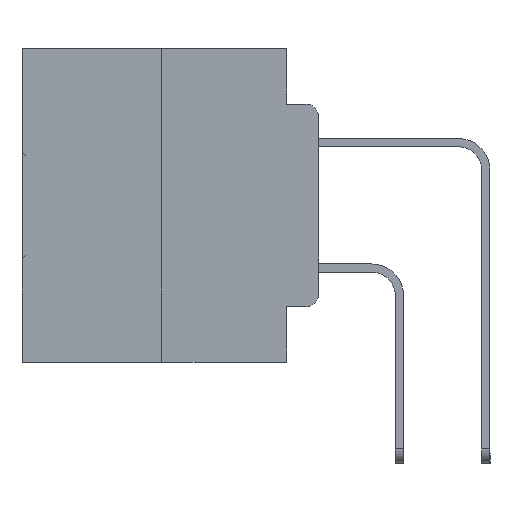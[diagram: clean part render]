
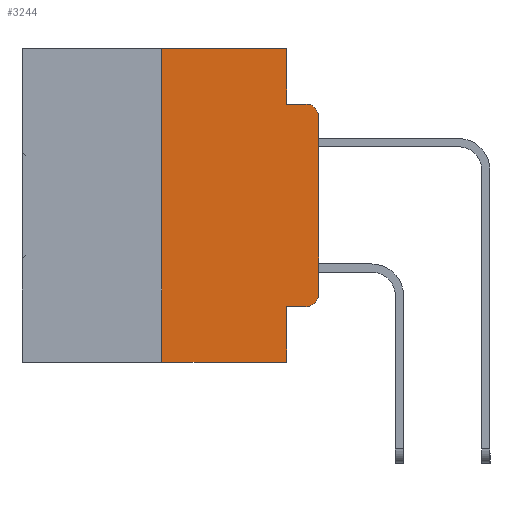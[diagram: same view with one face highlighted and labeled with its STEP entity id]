
A CAD part, left-side view. The second image highlights one B-rep face of the part: STEP entity #3244.
In plain terms, the highlighted planar face has unit normal (-1, 0, 0).
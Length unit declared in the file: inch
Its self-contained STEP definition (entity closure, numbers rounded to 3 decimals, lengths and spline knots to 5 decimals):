
#68 = EDGE_CURVE ( 'NONE', #25260, #1477, #29944, .T. ) ;
#420 = CARTESIAN_POINT ( 'NONE',  ( 0., 0.02, -0.1085 ) ) ;
#593 = CARTESIAN_POINT ( 'NONE',  ( 0., 0.25, 0. ) ) ;
#1342 = VECTOR ( 'NONE', #10830, 39.37008 ) ;
#1477 = VERTEX_POINT ( 'NONE', #18662 ) ;
#1720 = VERTEX_POINT ( 'NONE', #10265 ) ;
#2670 = VECTOR ( 'NONE', #6742, 39.37008 ) ;
#2685 = LINE ( 'NONE', #2778, #15886 ) ;
#2778 = CARTESIAN_POINT ( 'NONE',  ( 0., 0.473, 0. ) ) ;
#2793 = CARTESIAN_POINT ( 'NONE',  ( 0., 0.25, -0.5 ) ) ;
#3194 = CARTESIAN_POINT ( 'NONE',  ( 0., 0.25, 0. ) ) ;
#3244 = ADVANCED_FACE ( 'NONE', ( #16424 ), #9417, .F. ) ;
#3265 = DIRECTION ( 'NONE',  ( 0., 0., 1. ) ) ;
#3884 = VECTOR ( 'NONE', #8515, 39.37008 ) ;
#4052 = LINE ( 'NONE', #12203, #17966 ) ;
#4576 = AXIS2_PLACEMENT_3D ( 'NONE', #6762, #29817, #12055 ) ;
#4699 = DIRECTION ( 'NONE',  ( 0., 0., -1. ) ) ;
#4790 = VERTEX_POINT ( 'NONE', #2793 ) ;
#5269 = DIRECTION ( 'NONE',  ( 0., -1., 0. ) ) ;
#5430 = DIRECTION ( 'NONE',  ( -1., 0., 0. ) ) ;
#6102 = EDGE_CURVE ( 'NONE', #23875, #24633, #23472, .T. ) ;
#6383 = CARTESIAN_POINT ( 'NONE',  ( 0., 0.02, -0.3915 ) ) ;
#6742 = DIRECTION ( 'NONE',  ( 0., 0., -1. ) ) ;
#6762 = CARTESIAN_POINT ( 'NONE',  ( 0., 0.473, 0. ) ) ;
#7113 = ORIENTED_EDGE ( 'NONE', *, *, #7206, .T. ) ;
#7206 = EDGE_CURVE ( 'NONE', #1720, #25260, #32843, .T. ) ;
#8183 = CARTESIAN_POINT ( 'NONE',  ( 0., 0.051, 0. ) ) ;
#8515 = DIRECTION ( 'NONE',  ( 0., 0., 1. ) ) ;
#9063 = DIRECTION ( 'NONE',  ( 0., 0., -1. ) ) ;
#9417 = PLANE ( 'NONE',  #4576 ) ;
#9748 = DIRECTION ( 'NONE',  ( 0., -1., 0. ) ) ;
#9899 = CARTESIAN_POINT ( 'NONE',  ( 0., 0.051, -0.0885 ) ) ;
#9982 = CARTESIAN_POINT ( 'NONE',  ( 0., 0.051, 0. ) ) ;
#10265 = CARTESIAN_POINT ( 'NONE',  ( 0., 0., -0.3915 ) ) ;
#10830 = DIRECTION ( 'NONE',  ( 0., 0., -1. ) ) ;
#11194 = ORIENTED_EDGE ( 'NONE', *, *, #22410, .T. ) ;
#11533 = ORIENTED_EDGE ( 'NONE', *, *, #30102, .F. ) ;
#12055 = DIRECTION ( 'NONE',  ( 0., 0., -1. ) ) ;
#12203 = CARTESIAN_POINT ( 'NONE',  ( 0., 0.051, -0.0885 ) ) ;
#13129 = EDGE_CURVE ( 'NONE', #4790, #27835, #13350, .T. ) ;
#13208 = CIRCLE ( 'NONE', #30559, 0.02 ) ;
#13307 = ORIENTED_EDGE ( 'NONE', *, *, #68, .T. ) ;
#13350 = LINE ( 'NONE', #593, #19388 ) ;
#14724 = CARTESIAN_POINT ( 'NONE',  ( 0., 0., -0.1085 ) ) ;
#14835 = DIRECTION ( 'NONE',  ( 0., -1., 0. ) ) ;
#15886 = VECTOR ( 'NONE', #31241, 39.37008 ) ;
#16424 = FACE_OUTER_BOUND ( 'NONE', #30757, .T. ) ;
#16648 = EDGE_CURVE ( 'NONE', #24226, #19794, #28912, .T. ) ;
#17966 = VECTOR ( 'NONE', #14835, 39.37008 ) ;
#17997 = ORIENTED_EDGE ( 'NONE', *, *, #16648, .F. ) ;
#18026 = ORIENTED_EDGE ( 'NONE', *, *, #13129, .F. ) ;
#18305 = CARTESIAN_POINT ( 'NONE',  ( 0., 0.051, -0.4115 ) ) ;
#18471 = ORIENTED_EDGE ( 'NONE', *, *, #32550, .T. ) ;
#18662 = CARTESIAN_POINT ( 'NONE',  ( 0., 0.02, -0.0885 ) ) ;
#19388 = VECTOR ( 'NONE', #3265, 39.37008 ) ;
#19392 = CARTESIAN_POINT ( 'NONE',  ( 0., 0.02, -0.4115 ) ) ;
#19794 = VERTEX_POINT ( 'NONE', #9899 ) ;
#21504 = CARTESIAN_POINT ( 'NONE',  ( 0., 0.051, -0.4115 ) ) ;
#22410 = EDGE_CURVE ( 'NONE', #28571, #1720, #13208, .T. ) ;
#23472 = LINE ( 'NONE', #27486, #2670 ) ;
#23475 = EDGE_CURVE ( 'NONE', #19794, #1477, #4052, .T. ) ;
#23875 = VERTEX_POINT ( 'NONE', #21504 ) ;
#24049 = ORIENTED_EDGE ( 'NONE', *, *, #6102, .F. ) ;
#24226 = VERTEX_POINT ( 'NONE', #9982 ) ;
#24435 = ORIENTED_EDGE ( 'NONE', *, *, #30479, .T. ) ;
#24509 = DIRECTION ( 'NONE',  ( -1., 0., 0. ) ) ;
#24563 = CARTESIAN_POINT ( 'NONE',  ( 0., 0., 0. ) ) ;
#24633 = VERTEX_POINT ( 'NONE', #32528 ) ;
#25260 = VERTEX_POINT ( 'NONE', #14724 ) ;
#25857 = LINE ( 'NONE', #32647, #31762 ) ;
#27486 = CARTESIAN_POINT ( 'NONE',  ( 0., 0.051, 0. ) ) ;
#27835 = VERTEX_POINT ( 'NONE', #3194 ) ;
#28571 = VERTEX_POINT ( 'NONE', #19392 ) ;
#28912 = LINE ( 'NONE', #8183, #1342 ) ;
#29817 = DIRECTION ( 'NONE',  ( 1., 0., 0. ) ) ;
#29944 = CIRCLE ( 'NONE', #31883, 0.02 ) ;
#30102 = EDGE_CURVE ( 'NONE', #27835, #24226, #2685, .T. ) ;
#30479 = EDGE_CURVE ( 'NONE', #4790, #24633, #25857, .T. ) ;
#30559 = AXIS2_PLACEMENT_3D ( 'NONE', #6383, #24509, #9063 ) ;
#30757 = EDGE_LOOP ( 'NONE', ( #7113, #13307, #31451, #17997, #11533, #18026, #24435, #24049, #18471, #11194 ) ) ;
#31241 = DIRECTION ( 'NONE',  ( 0., -1., 0. ) ) ;
#31451 = ORIENTED_EDGE ( 'NONE', *, *, #23475, .F. ) ;
#31762 = VECTOR ( 'NONE', #9748, 39.37008 ) ;
#31883 = AXIS2_PLACEMENT_3D ( 'NONE', #420, #5430, #4699 ) ;
#32462 = LINE ( 'NONE', #18305, #33144 ) ;
#32528 = CARTESIAN_POINT ( 'NONE',  ( 0., 0.051, -0.5 ) ) ;
#32550 = EDGE_CURVE ( 'NONE', #23875, #28571, #32462, .T. ) ;
#32647 = CARTESIAN_POINT ( 'NONE',  ( 0., 0.473, -0.5 ) ) ;
#32843 = LINE ( 'NONE', #24563, #3884 ) ;
#33144 = VECTOR ( 'NONE', #5269, 39.37008 ) ;
